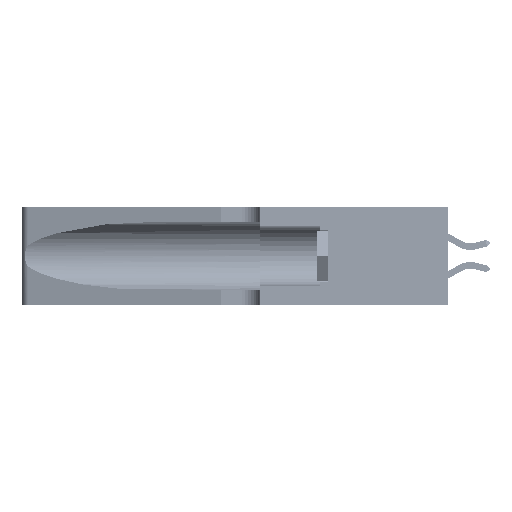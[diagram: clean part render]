
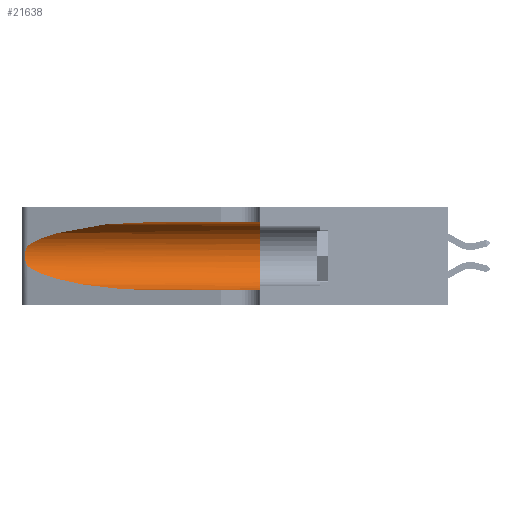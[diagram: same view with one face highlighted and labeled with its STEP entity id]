
A CAD part, left-side view. The second image highlights one B-rep face of the part: STEP entity #21638.
In plain terms, the highlighted cylindrical face has radius 3.308 mm (diameter 6.617 mm), a partial arc.
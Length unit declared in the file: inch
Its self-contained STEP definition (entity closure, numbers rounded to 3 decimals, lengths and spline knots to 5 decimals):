
#142 = ORIENTED_EDGE ( 'NONE', *, *, #33938, .T. ) ;
#366 =( BOUNDED_CURVE ( )  B_SPLINE_CURVE ( 3, ( #43586, #36365, #4123, #29277 ),
 .UNSPECIFIED., .F., .T. ) 
 B_SPLINE_CURVE_WITH_KNOTS ( ( 4, 4 ),
 ( 3.44316, 4.71239 ),
 .UNSPECIFIED. ) 
 CURVE ( )  GEOMETRIC_REPRESENTATION_ITEM ( )  RATIONAL_B_SPLINE_CURVE ( ( 1., 0.87, 0.87, 1. ) ) 
 REPRESENTATION_ITEM ( '' )  );
#369 = CARTESIAN_POINT ( 'NONE',  ( 0.26075, 1.23896, 0.19203 ) ) ;
#812 = ORIENTED_EDGE ( 'NONE', *, *, #5208, .T. ) ;
#1150 = AXIS2_PLACEMENT_3D ( 'NONE', #9189, #34354, #12801 ) ;
#1351 = CARTESIAN_POINT ( 'NONE',  ( 0.25487, 1.22718, 0.22369 ) ) ;
#2503 = ORIENTED_EDGE ( 'NONE', *, *, #25490, .F. ) ;
#3951 = CARTESIAN_POINT ( 'NONE',  ( 0.26017, 1.23833, 0.17102 ) ) ;
#4123 = CARTESIAN_POINT ( 'NONE',  ( 0.18966, 0.96281, 0.05475 ) ) ;
#4419 = ORIENTED_EDGE ( 'NONE', *, *, #45042, .T. ) ;
#5208 = EDGE_CURVE ( 'NONE', #9210, #37291, #37262, .T. ) ;
#5246 =( BOUNDED_CURVE ( )  B_SPLINE_CURVE ( 3, ( #22676, #19213, #30074, #8518 ),
 .UNSPECIFIED., .F., .F. ) 
 B_SPLINE_CURVE_WITH_KNOTS ( ( 4, 4 ),
 ( 1.5708, 2.84003 ),
 .UNSPECIFIED. ) 
 CURVE ( )  GEOMETRIC_REPRESENTATION_ITEM ( )  RATIONAL_B_SPLINE_CURVE ( ( 1., 0.87, 0.87, 1. ) ) 
 REPRESENTATION_ITEM ( '' )  );
#5470 = DIRECTION ( 'NONE',  ( 0., 0., -1. ) ) ;
#7583 = CARTESIAN_POINT ( 'NONE',  ( 0.25789, 1.23486, 0.15765 ) ) ;
#8339 = LINE ( 'NONE', #26559, #25196 ) ;
#8518 = CARTESIAN_POINT ( 'NONE',  ( 0.25487, 1.22718, 0.22369 ) ) ;
#9189 = CARTESIAN_POINT ( 'NONE',  ( 0.1305, 0.35, 0.185 ) ) ;
#9210 = VERTEX_POINT ( 'NONE', #1351 ) ;
#10743 = VERTEX_POINT ( 'NONE', #19405 ) ;
#11169 = CARTESIAN_POINT ( 'NONE',  ( 0.25555, 1.22993, 0.14849 ) ) ;
#12419 = DIRECTION ( 'NONE',  ( 0., -1., 0. ) ) ;
#12635 = VERTEX_POINT ( 'NONE', #40988 ) ;
#12801 = DIRECTION ( 'NONE',  ( 0., 0., 1. ) ) ;
#12882 = VECTOR ( 'NONE', #46481, 39.37008 ) ;
#13750 = FACE_OUTER_BOUND ( 'NONE', #39704, .T. ) ;
#14668 = CARTESIAN_POINT ( 'NONE',  ( 0.25555, 1.22994, 0.2215 ) ) ;
#18258 = CARTESIAN_POINT ( 'NONE',  ( 0.25787, 1.23484, 0.2124 ) ) ;
#19213 = CARTESIAN_POINT ( 'NONE',  ( 0.18966, 0.96281, 0.31525 ) ) ;
#19405 = CARTESIAN_POINT ( 'NONE',  ( 0.1305, 0.35, 0.31525 ) ) ;
#19544 = EDGE_CURVE ( 'NONE', #12635, #20556, #8339, .T. ) ;
#20556 = VERTEX_POINT ( 'NONE', #36257 ) ;
#21318 = LINE ( 'NONE', #21323, #12882 ) ;
#21323 = CARTESIAN_POINT ( 'NONE',  ( 0.1305, 1.61858, 0.31525 ) ) ;
#21638 = ADVANCED_FACE ( 'NONE', ( #13750 ), #31776, .F. ) ;
#21865 = CARTESIAN_POINT ( 'NONE',  ( 0.26018, 1.23835, 0.19895 ) ) ;
#22676 = CARTESIAN_POINT ( 'NONE',  ( 0.1305, 0.72297, 0.31525 ) ) ;
#24055 = ORIENTED_EDGE ( 'NONE', *, *, #25053, .F. ) ;
#25053 = EDGE_CURVE ( 'NONE', #37263, #10743, #21318, .T. ) ;
#25196 = VECTOR ( 'NONE', #12419, 39.37008 ) ;
#25486 = CARTESIAN_POINT ( 'NONE',  ( 0.26075, 1.23896, 0.178 ) ) ;
#25490 = EDGE_CURVE ( 'NONE', #10743, #20556, #43795, .T. ) ;
#26559 = CARTESIAN_POINT ( 'NONE',  ( 0.1305, 1.61858, 0.05475 ) ) ;
#27812 = CARTESIAN_POINT ( 'NONE',  ( 0.1305, 0.72297, 0.31525 ) ) ;
#29124 = CARTESIAN_POINT ( 'NONE',  ( 0.25856, 1.23593, 0.16098 ) ) ;
#29277 = CARTESIAN_POINT ( 'NONE',  ( 0.1305, 0.72297, 0.05475 ) ) ;
#30074 = CARTESIAN_POINT ( 'NONE',  ( 0.2373, 1.15595, 0.28018 ) ) ;
#31776 = CYLINDRICAL_SURFACE ( 'NONE', #33595, 0.13025 ) ;
#32588 = CARTESIAN_POINT ( 'NONE',  ( 0.25639, 1.23184, 0.21858 ) ) ;
#32757 = CARTESIAN_POINT ( 'NONE',  ( 0.25639, 1.23186, 0.15144 ) ) ;
#33595 = AXIS2_PLACEMENT_3D ( 'NONE', #34240, #37880, #5470 ) ;
#33938 = EDGE_CURVE ( 'NONE', #37291, #12635, #366, .T. ) ;
#34240 = CARTESIAN_POINT ( 'NONE',  ( 0.1305, 1.61858, 0.185 ) ) ;
#34354 = DIRECTION ( 'NONE',  ( 0., 1., 0. ) ) ;
#36257 = CARTESIAN_POINT ( 'NONE',  ( 0.1305, 0.35, 0.05475 ) ) ;
#36365 = CARTESIAN_POINT ( 'NONE',  ( 0.2373, 1.15595, 0.08982 ) ) ;
#36367 = CARTESIAN_POINT ( 'NONE',  ( 0.25487, 1.22718, 0.14631 ) ) ;
#37262 = B_SPLINE_CURVE_WITH_KNOTS ( 'NONE', 3,
 ( #39829, #14668, #32588, #18258, #43432, #21865, #369, #25486, #3951, #29124, #7583, #32757, #11169, #36367 ),
 .UNSPECIFIED., .F., .F.,
 ( 4, 2, 2, 2, 2, 2, 4 ),
 ( 0., 0.00027, 0.00053, 0.00107, 0.0016, 0.00187, 0.00214 ),
 .UNSPECIFIED. ) ;
#37263 = VERTEX_POINT ( 'NONE', #27812 ) ;
#37291 = VERTEX_POINT ( 'NONE', #38670 ) ;
#37516 = ORIENTED_EDGE ( 'NONE', *, *, #19544, .T. ) ;
#37880 = DIRECTION ( 'NONE',  ( 0., -1., 0. ) ) ;
#38670 = CARTESIAN_POINT ( 'NONE',  ( 0.25487, 1.22718, 0.14631 ) ) ;
#39704 = EDGE_LOOP ( 'NONE', ( #4419, #812, #142, #37516, #2503, #24055 ) ) ;
#39829 = CARTESIAN_POINT ( 'NONE',  ( 0.25487, 1.22718, 0.22369 ) ) ;
#40988 = CARTESIAN_POINT ( 'NONE',  ( 0.1305, 0.72297, 0.05475 ) ) ;
#43432 = CARTESIAN_POINT ( 'NONE',  ( 0.25854, 1.2359, 0.20912 ) ) ;
#43586 = CARTESIAN_POINT ( 'NONE',  ( 0.25487, 1.22718, 0.14631 ) ) ;
#43795 = CIRCLE ( 'NONE', #1150, 0.13025 ) ;
#45042 = EDGE_CURVE ( 'NONE', #37263, #9210, #5246, .T. ) ;
#46481 = DIRECTION ( 'NONE',  ( 0., -1., 0. ) ) ;
